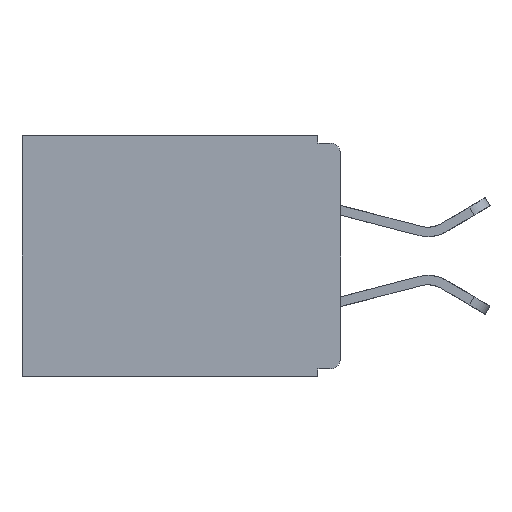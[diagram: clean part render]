
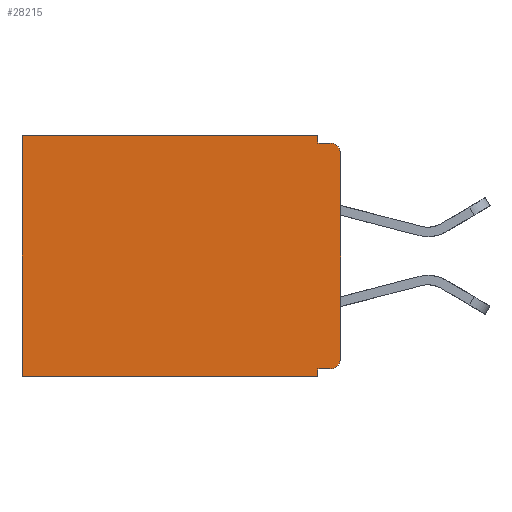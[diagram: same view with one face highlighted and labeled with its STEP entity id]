
A CAD part, left-side view. The second image highlights one B-rep face of the part: STEP entity #28215.
In plain terms, the highlighted planar face has unit normal (-1, 0, 0).
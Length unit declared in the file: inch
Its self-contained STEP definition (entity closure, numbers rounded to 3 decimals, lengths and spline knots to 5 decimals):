
#176 = EDGE_CURVE ( 'NONE', #2239, #8236, #25420, .T. ) ;
#522 = CARTESIAN_POINT ( 'NONE',  ( 0.3, 0.015, -0.025 ) ) ;
#1067 = CARTESIAN_POINT ( 'NONE',  ( 0.3, 0.437, -0.33 ) ) ;
#1206 = VERTEX_POINT ( 'NONE', #14803 ) ;
#1408 = LINE ( 'NONE', #26585, #25859 ) ;
#2138 = CIRCLE ( 'NONE', #8979, 0.015 ) ;
#2239 = VERTEX_POINT ( 'NONE', #11551 ) ;
#2524 = AXIS2_PLACEMENT_3D ( 'NONE', #15735, #3828, #20520 ) ;
#2870 = DIRECTION ( 'NONE',  ( 0., 0., -1. ) ) ;
#2976 = VECTOR ( 'NONE', #18898, 39.37008 ) ;
#3828 = DIRECTION ( 'NONE',  ( 1., 0., 0. ) ) ;
#4219 = VERTEX_POINT ( 'NONE', #11613 ) ;
#4464 = VERTEX_POINT ( 'NONE', #28822 ) ;
#5156 = ORIENTED_EDGE ( 'NONE', *, *, #14532, .F. ) ;
#5374 = CARTESIAN_POINT ( 'NONE',  ( 0.3, 0.031, 0. ) ) ;
#6555 = DIRECTION ( 'NONE',  ( -1., 0., 0. ) ) ;
#6563 = LINE ( 'NONE', #13504, #18558 ) ;
#6951 = EDGE_CURVE ( 'NONE', #30466, #23049, #22004, .T. ) ;
#8065 = DIRECTION ( 'NONE',  ( 0., 0., -1. ) ) ;
#8236 = VERTEX_POINT ( 'NONE', #13109 ) ;
#8402 = CARTESIAN_POINT ( 'NONE',  ( 0.3, 0.031, -0.32 ) ) ;
#8979 = AXIS2_PLACEMENT_3D ( 'NONE', #522, #17197, #2870 ) ;
#9024 = VECTOR ( 'NONE', #28864, 39.37008 ) ;
#9277 = ORIENTED_EDGE ( 'NONE', *, *, #23695, .F. ) ;
#9473 = EDGE_CURVE ( 'NONE', #23049, #4219, #9704, .T. ) ;
#9501 = ORIENTED_EDGE ( 'NONE', *, *, #22753, .T. ) ;
#9638 = ORIENTED_EDGE ( 'NONE', *, *, #9473, .T. ) ;
#9704 = LINE ( 'NONE', #1067, #28546 ) ;
#10364 = VERTEX_POINT ( 'NONE', #23172 ) ;
#10824 = DIRECTION ( 'NONE',  ( 0., 1., 0. ) ) ;
#10993 = ORIENTED_EDGE ( 'NONE', *, *, #23985, .F. ) ;
#11334 = EDGE_CURVE ( 'NONE', #24046, #4219, #24114, .T. ) ;
#11473 = VECTOR ( 'NONE', #10824, 39.37008 ) ;
#11551 = CARTESIAN_POINT ( 'NONE',  ( 0.3, 0., -0.025 ) ) ;
#11613 = CARTESIAN_POINT ( 'NONE',  ( 0.3, 0.437, -0.33 ) ) ;
#12279 = EDGE_CURVE ( 'NONE', #30466, #4464, #16306, .T. ) ;
#13109 = CARTESIAN_POINT ( 'NONE',  ( 0.3, 0., -0.305 ) ) ;
#13504 = CARTESIAN_POINT ( 'NONE',  ( 0.3, 0., -0.32 ) ) ;
#14532 = EDGE_CURVE ( 'NONE', #29984, #24046, #20260, .T. ) ;
#14803 = CARTESIAN_POINT ( 'NONE',  ( 0.3, 0.015, -0.01 ) ) ;
#14810 = CARTESIAN_POINT ( 'NONE',  ( 0.3, 0.031, -0.33 ) ) ;
#14891 = CARTESIAN_POINT ( 'NONE',  ( 0.3, 0., -0.33 ) ) ;
#15735 = CARTESIAN_POINT ( 'NONE',  ( 0.3, 0., -0.33 ) ) ;
#16306 = LINE ( 'NONE', #25971, #21879 ) ;
#16799 = ORIENTED_EDGE ( 'NONE', *, *, #6951, .T. ) ;
#17197 = DIRECTION ( 'NONE',  ( -1., 0., 0. ) ) ;
#17763 = DIRECTION ( 'NONE',  ( 0., 0., -1. ) ) ;
#18313 = DIRECTION ( 'NONE',  ( 0., 1., 0. ) ) ;
#18499 = VECTOR ( 'NONE', #8065, 39.37008 ) ;
#18558 = VECTOR ( 'NONE', #18313, 39.37008 ) ;
#18816 = AXIS2_PLACEMENT_3D ( 'NONE', #20883, #6555, #23229 ) ;
#18868 = CARTESIAN_POINT ( 'NONE',  ( 0.3, 0., 0. ) ) ;
#18898 = DIRECTION ( 'NONE',  ( 0., 1., 0. ) ) ;
#19375 = ORIENTED_EDGE ( 'NONE', *, *, #11334, .F. ) ;
#19788 = EDGE_LOOP ( 'NONE', ( #26317, #24853, #9277, #20497, #16799, #9638, #19375, #5156, #10993, #9501 ) ) ;
#20260 = LINE ( 'NONE', #14810, #9024 ) ;
#20352 = CARTESIAN_POINT ( 'NONE',  ( 0.3, 0., -0.33 ) ) ;
#20497 = ORIENTED_EDGE ( 'NONE', *, *, #12279, .F. ) ;
#20520 = DIRECTION ( 'NONE',  ( 0., 0., -1. ) ) ;
#20883 = CARTESIAN_POINT ( 'NONE',  ( 0.3, 0.015, -0.305 ) ) ;
#20910 = CARTESIAN_POINT ( 'NONE',  ( 0.3, 0.031, -0.33 ) ) ;
#21879 = VECTOR ( 'NONE', #23687, 39.37008 ) ;
#21945 = DIRECTION ( 'NONE',  ( 0., -1., 0. ) ) ;
#22004 = LINE ( 'NONE', #18868, #2976 ) ;
#22753 = EDGE_CURVE ( 'NONE', #10364, #8236, #29568, .T. ) ;
#23049 = VERTEX_POINT ( 'NONE', #26525 ) ;
#23172 = CARTESIAN_POINT ( 'NONE',  ( 0.3, 0.015, -0.32 ) ) ;
#23206 = FACE_OUTER_BOUND ( 'NONE', #19788, .T. ) ;
#23229 = DIRECTION ( 'NONE',  ( 0., 0., -1. ) ) ;
#23669 = EDGE_CURVE ( 'NONE', #2239, #1206, #2138, .T. ) ;
#23687 = DIRECTION ( 'NONE',  ( 0., 0., -1. ) ) ;
#23695 = EDGE_CURVE ( 'NONE', #4464, #1206, #1408, .T. ) ;
#23985 = EDGE_CURVE ( 'NONE', #10364, #29984, #6563, .T. ) ;
#24046 = VERTEX_POINT ( 'NONE', #20910 ) ;
#24114 = LINE ( 'NONE', #20352, #11473 ) ;
#24853 = ORIENTED_EDGE ( 'NONE', *, *, #23669, .T. ) ;
#25420 = LINE ( 'NONE', #14891, #18499 ) ;
#25859 = VECTOR ( 'NONE', #21945, 39.37008 ) ;
#25971 = CARTESIAN_POINT ( 'NONE',  ( 0.3, 0.031, 0. ) ) ;
#26317 = ORIENTED_EDGE ( 'NONE', *, *, #176, .F. ) ;
#26525 = CARTESIAN_POINT ( 'NONE',  ( 0.3, 0.437, 0. ) ) ;
#26585 = CARTESIAN_POINT ( 'NONE',  ( 0.3, 0., -0.01 ) ) ;
#27416 = PLANE ( 'NONE',  #2524 ) ;
#28215 = ADVANCED_FACE ( 'NONE', ( #23206 ), #27416, .F. ) ;
#28546 = VECTOR ( 'NONE', #17763, 39.37008 ) ;
#28822 = CARTESIAN_POINT ( 'NONE',  ( 0.3, 0.031, -0.01 ) ) ;
#28864 = DIRECTION ( 'NONE',  ( 0., 0., -1. ) ) ;
#29568 = CIRCLE ( 'NONE', #18816, 0.015 ) ;
#29984 = VERTEX_POINT ( 'NONE', #8402 ) ;
#30466 = VERTEX_POINT ( 'NONE', #5374 ) ;
